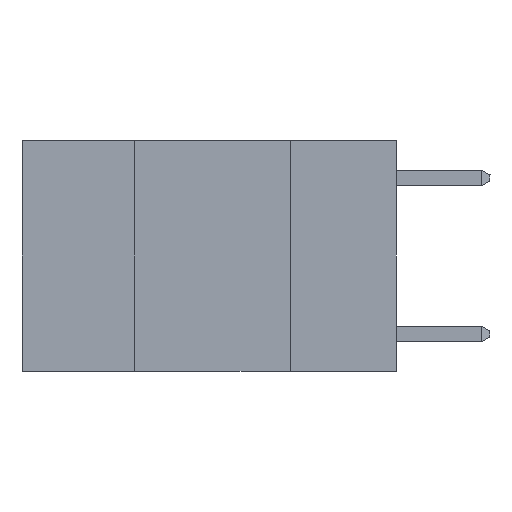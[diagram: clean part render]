
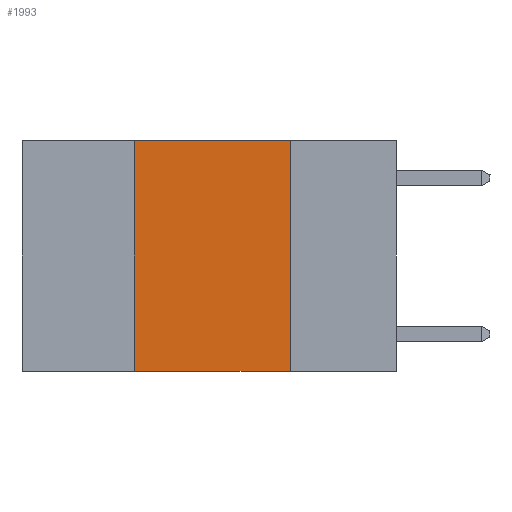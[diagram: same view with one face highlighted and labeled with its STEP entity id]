
A CAD part, left-side view. The second image highlights one B-rep face of the part: STEP entity #1993.
In plain terms, the highlighted planar face has unit normal (-1, 0, 0).
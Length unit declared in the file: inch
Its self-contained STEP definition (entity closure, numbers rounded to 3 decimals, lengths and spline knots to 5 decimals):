
#1257 = LINE ( 'NONE', #7079, #5038 ) ;
#1658 = EDGE_CURVE ( 'NONE', #6810, #3169, #1257, .T. ) ;
#1993 = ADVANCED_FACE ( 'NONE', ( #13039 ), #5093, .F. ) ;
#2252 = CARTESIAN_POINT ( 'NONE',  ( 0., 0.42, 0. ) ) ;
#2336 = VECTOR ( 'NONE', #11914, 39.37008 ) ;
#2374 = CARTESIAN_POINT ( 'NONE',  ( 0., 0.42, -0.37 ) ) ;
#2661 = AXIS2_PLACEMENT_3D ( 'NONE', #12154, #13103, #7152 ) ;
#3169 = VERTEX_POINT ( 'NONE', #2252 ) ;
#4021 = VERTEX_POINT ( 'NONE', #8682 ) ;
#4901 = VECTOR ( 'NONE', #8669, 39.37008 ) ;
#5038 = VECTOR ( 'NONE', #11112, 39.37008 ) ;
#5093 = PLANE ( 'NONE',  #2661 ) ;
#5299 = LINE ( 'NONE', #7920, #2336 ) ;
#6810 = VERTEX_POINT ( 'NONE', #2374 ) ;
#7029 = LINE ( 'NONE', #8694, #9389 ) ;
#7079 = CARTESIAN_POINT ( 'NONE',  ( 0., 0.42, 0. ) ) ;
#7152 = DIRECTION ( 'NONE',  ( 0., 0., -1. ) ) ;
#7606 = VERTEX_POINT ( 'NONE', #9753 ) ;
#7920 = CARTESIAN_POINT ( 'NONE',  ( 0., 0.17, 0. ) ) ;
#8669 = DIRECTION ( 'NONE',  ( 0., -1., 0. ) ) ;
#8682 = CARTESIAN_POINT ( 'NONE',  ( 0., 0.17, 0. ) ) ;
#8694 = CARTESIAN_POINT ( 'NONE',  ( 0., 0.6, -0.37 ) ) ;
#9389 = VECTOR ( 'NONE', #12682, 39.37008 ) ;
#9507 = EDGE_CURVE ( 'NONE', #4021, #7606, #5299, .T. ) ;
#9753 = CARTESIAN_POINT ( 'NONE',  ( 0., 0.17, -0.37 ) ) ;
#10133 = EDGE_CURVE ( 'NONE', #6810, #7606, #7029, .T. ) ;
#10149 = ORIENTED_EDGE ( 'NONE', *, *, #9507, .F. ) ;
#10290 = EDGE_LOOP ( 'NONE', ( #10149, #10297, #11388, #12404 ) ) ;
#10297 = ORIENTED_EDGE ( 'NONE', *, *, #11891, .F. ) ;
#10324 = LINE ( 'NONE', #13572, #4901 ) ;
#11112 = DIRECTION ( 'NONE',  ( 0., 0., 1. ) ) ;
#11388 = ORIENTED_EDGE ( 'NONE', *, *, #1658, .F. ) ;
#11891 = EDGE_CURVE ( 'NONE', #3169, #4021, #10324, .T. ) ;
#11914 = DIRECTION ( 'NONE',  ( 0., 0., -1. ) ) ;
#12154 = CARTESIAN_POINT ( 'NONE',  ( 0., 0.6, 0. ) ) ;
#12404 = ORIENTED_EDGE ( 'NONE', *, *, #10133, .T. ) ;
#12682 = DIRECTION ( 'NONE',  ( 0., -1., 0. ) ) ;
#13039 = FACE_OUTER_BOUND ( 'NONE', #10290, .T. ) ;
#13103 = DIRECTION ( 'NONE',  ( 1., 0., 0. ) ) ;
#13572 = CARTESIAN_POINT ( 'NONE',  ( 0., 0.6, 0. ) ) ;
